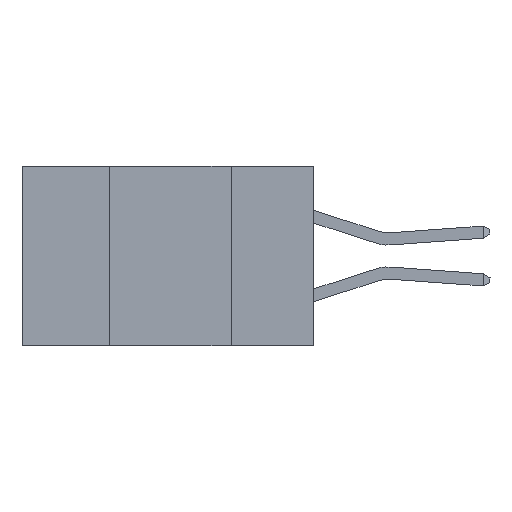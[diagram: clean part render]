
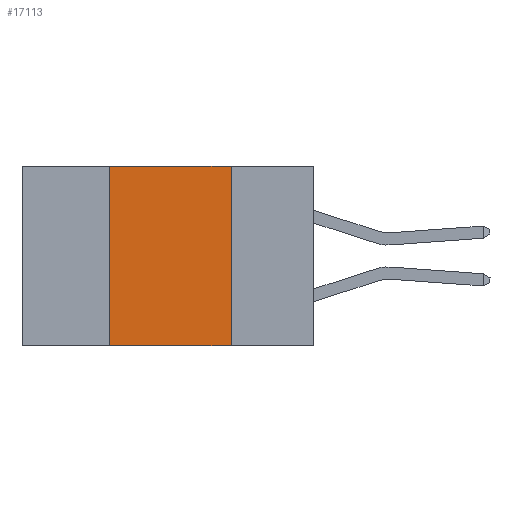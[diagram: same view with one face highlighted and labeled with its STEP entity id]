
A CAD part, left-side view. The second image highlights one B-rep face of the part: STEP entity #17113.
In plain terms, the highlighted planar face has unit normal (-1, 0, 0).
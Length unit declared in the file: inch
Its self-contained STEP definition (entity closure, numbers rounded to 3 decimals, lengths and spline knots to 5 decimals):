
#1068 = CARTESIAN_POINT ( 'NONE',  ( 0., 0.42, -0.37 ) ) ;
#2245 = ORIENTED_EDGE ( 'NONE', *, *, #2789, .F. ) ;
#2789 = EDGE_CURVE ( 'NONE', #9870, #26857, #14773, .T. ) ;
#6859 = VECTOR ( 'NONE', #27366, 39.37008 ) ;
#6972 = EDGE_CURVE ( 'NONE', #25488, #17118, #24484, .T. ) ;
#7271 = DIRECTION ( 'NONE',  ( 0., -1., 0. ) ) ;
#7778 = ORIENTED_EDGE ( 'NONE', *, *, #11007, .T. ) ;
#8407 = CARTESIAN_POINT ( 'NONE',  ( 0., 0.6, -0.37 ) ) ;
#8683 = DIRECTION ( 'NONE',  ( 0., 0., -1. ) ) ;
#9870 = VERTEX_POINT ( 'NONE', #1068 ) ;
#10840 = VECTOR ( 'NONE', #15676, 39.37008 ) ;
#11007 = EDGE_CURVE ( 'NONE', #9870, #17118, #23409, .T. ) ;
#11280 = AXIS2_PLACEMENT_3D ( 'NONE', #23416, #25797, #8683 ) ;
#11785 = ORIENTED_EDGE ( 'NONE', *, *, #15899, .F. ) ;
#12375 = FACE_OUTER_BOUND ( 'NONE', #25432, .T. ) ;
#14773 = LINE ( 'NONE', #25106, #6859 ) ;
#15676 = DIRECTION ( 'NONE',  ( 0., 0., -1. ) ) ;
#15899 = EDGE_CURVE ( 'NONE', #26857, #25488, #20036, .T. ) ;
#15912 = ORIENTED_EDGE ( 'NONE', *, *, #6972, .F. ) ;
#17104 = DIRECTION ( 'NONE',  ( 0., -1., 0. ) ) ;
#17113 = ADVANCED_FACE ( 'NONE', ( #12375 ), #20917, .F. ) ;
#17118 = VERTEX_POINT ( 'NONE', #19078 ) ;
#18042 = CARTESIAN_POINT ( 'NONE',  ( 0., 0.17, 0. ) ) ;
#18218 = VECTOR ( 'NONE', #17104, 39.37008 ) ;
#19078 = CARTESIAN_POINT ( 'NONE',  ( 0., 0.17, -0.37 ) ) ;
#20007 = CARTESIAN_POINT ( 'NONE',  ( 0., 0.17, 0. ) ) ;
#20036 = LINE ( 'NONE', #24239, #26480 ) ;
#20576 = CARTESIAN_POINT ( 'NONE',  ( 0., 0.42, 0. ) ) ;
#20917 = PLANE ( 'NONE',  #11280 ) ;
#23409 = LINE ( 'NONE', #8407, #18218 ) ;
#23416 = CARTESIAN_POINT ( 'NONE',  ( 0., 0.6, 0. ) ) ;
#24239 = CARTESIAN_POINT ( 'NONE',  ( 0., 0.6, 0. ) ) ;
#24484 = LINE ( 'NONE', #20007, #10840 ) ;
#25106 = CARTESIAN_POINT ( 'NONE',  ( 0., 0.42, 0. ) ) ;
#25432 = EDGE_LOOP ( 'NONE', ( #15912, #11785, #2245, #7778 ) ) ;
#25488 = VERTEX_POINT ( 'NONE', #18042 ) ;
#25797 = DIRECTION ( 'NONE',  ( 1., 0., 0. ) ) ;
#26480 = VECTOR ( 'NONE', #7271, 39.37008 ) ;
#26857 = VERTEX_POINT ( 'NONE', #20576 ) ;
#27366 = DIRECTION ( 'NONE',  ( 0., 0., 1. ) ) ;
